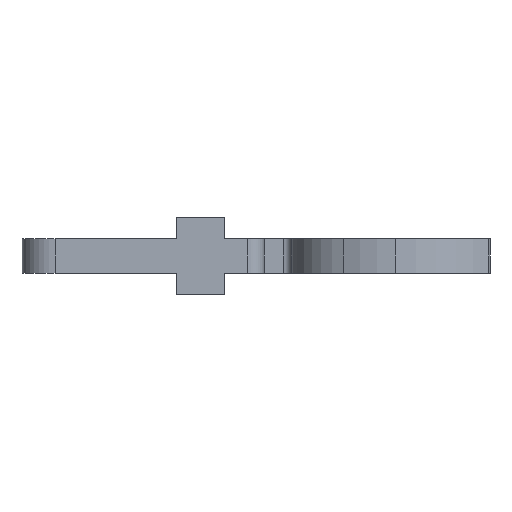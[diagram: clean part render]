
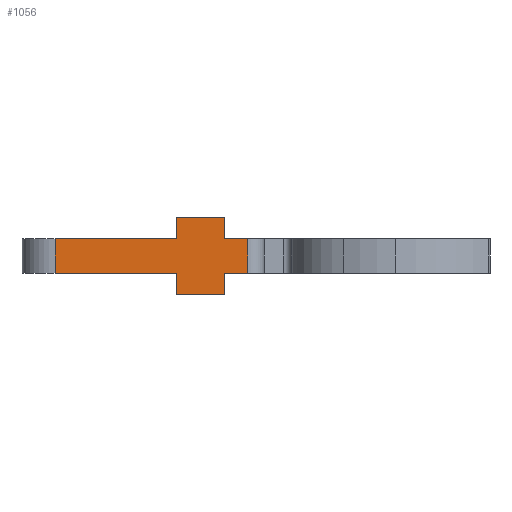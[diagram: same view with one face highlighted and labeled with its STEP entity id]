
A CAD part, left-side view. The second image highlights one B-rep face of the part: STEP entity #1056.
In plain terms, the highlighted planar face has unit normal (-1, 0, 0).
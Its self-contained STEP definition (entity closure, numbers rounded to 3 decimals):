
#2 = LINE ( 'NONE', #1489, #1785 ) ;
#8 = VERTEX_POINT ( 'NONE', #1669 ) ;
#20 = VERTEX_POINT ( 'NONE', #1665 ) ;
#34 = VERTEX_POINT ( 'NONE', #1617 ) ;
#60 = LINE ( 'NONE', #1410, #756 ) ;
#91 = LINE ( 'NONE', #1446, #873 ) ;
#95 = LINE ( 'NONE', #1477, #1276 ) ;
#170 = LINE ( 'NONE', #390, #1345 ) ;
#235 = LINE ( 'NONE', #439, #650 ) ;
#284 = EDGE_CURVE ( 'NONE', #642, #856, #235, .T. ) ;
#305 = EDGE_CURVE ( 'NONE', #1772, #20, #170, .T. ) ;
#320 = DIRECTION ( 'NONE',  ( 0., -1., 0. ) ) ;
#344 = VECTOR ( 'NONE', #1428, 1000. ) ;
#347 = VERTEX_POINT ( 'NONE', #1782 ) ;
#359 = EDGE_CURVE ( 'NONE', #765, #8, #903, .T. ) ;
#377 = VECTOR ( 'NONE', #1806, 1000. ) ;
#390 = CARTESIAN_POINT ( 'NONE',  ( 0., 23.241, 0. ) ) ;
#391 = CARTESIAN_POINT ( 'NONE',  ( 0., 20.066, 0. ) ) ;
#400 = LINE ( 'NONE', #1427, #817 ) ;
#413 = CARTESIAN_POINT ( 'NONE',  ( 0., 8.382, 3.302 ) ) ;
#439 = CARTESIAN_POINT ( 'NONE',  ( 0., 23.241, 0. ) ) ;
#441 = CARTESIAN_POINT ( 'NONE',  ( 0., 3.81, 5.334 ) ) ;
#468 = DIRECTION ( 'NONE',  ( 0., -1., 0. ) ) ;
#540 = EDGE_CURVE ( 'NONE', #856, #8, #1574, .T. ) ;
#547 = EDGE_CURVE ( 'NONE', #1663, #765, #2, .T. ) ;
#548 = EDGE_CURVE ( 'NONE', #1128, #1663, #95, .T. ) ;
#556 = EDGE_CURVE ( 'NONE', #1128, #1730, #91, .T. ) ;
#561 = EDGE_CURVE ( 'NONE', #34, #1730, #1613, .T. ) ;
#580 = EDGE_CURVE ( 'NONE', #34, #1772, #400, .T. ) ;
#583 = EDGE_CURVE ( 'NONE', #347, #20, #60, .T. ) ;
#589 = EDGE_CURVE ( 'NONE', #1293, #347, #1566, .T. ) ;
#592 = CARTESIAN_POINT ( 'NONE',  ( 0., 3.81, -2.032 ) ) ;
#593 = EDGE_CURVE ( 'NONE', #1293, #642, #1229, .T. ) ;
#642 = VERTEX_POINT ( 'NONE', #1357 ) ;
#650 = VECTOR ( 'NONE', #468, 1000. ) ;
#677 = CARTESIAN_POINT ( 'NONE',  ( 0., 8.382, 5.334 ) ) ;
#700 = DIRECTION ( 'NONE',  ( 0., 1., 0. ) ) ;
#704 = CARTESIAN_POINT ( 'NONE',  ( 0., 23.241, 3.302 ) ) ;
#714 = ORIENTED_EDGE ( 'NONE', *, *, #305, .T. ) ;
#718 = ORIENTED_EDGE ( 'NONE', *, *, #589, .F. ) ;
#729 = DIRECTION ( 'NONE',  ( 1., 0., 0. ) ) ;
#752 = PLANE ( 'NONE',  #1766 ) ;
#756 = VECTOR ( 'NONE', #1404, 1000. ) ;
#765 = VERTEX_POINT ( 'NONE', #1174 ) ;
#802 = ORIENTED_EDGE ( 'NONE', *, *, #580, .T. ) ;
#803 = ORIENTED_EDGE ( 'NONE', *, *, #561, .F. ) ;
#817 = VECTOR ( 'NONE', #1444, 1000. ) ;
#856 = VERTEX_POINT ( 'NONE', #997 ) ;
#873 = VECTOR ( 'NONE', #1457, 1000. ) ;
#903 = LINE ( 'NONE', #1817, #377 ) ;
#997 = CARTESIAN_POINT ( 'NONE',  ( 0., 1.587, 0. ) ) ;
#1007 = ORIENTED_EDGE ( 'NONE', *, *, #583, .F. ) ;
#1013 = FACE_OUTER_BOUND ( 'NONE', #1508, .T. ) ;
#1056 = ADVANCED_FACE ( 'NONE', ( #1013 ), #752, .F. ) ;
#1079 = ORIENTED_EDGE ( 'NONE', *, *, #593, .T. ) ;
#1107 = ORIENTED_EDGE ( 'NONE', *, *, #540, .T. ) ;
#1128 = VERTEX_POINT ( 'NONE', #677 ) ;
#1174 = CARTESIAN_POINT ( 'NONE',  ( 0., 3.81, 3.302 ) ) ;
#1184 = VECTOR ( 'NONE', #1396, 1000. ) ;
#1229 = LINE ( 'NONE', #1409, #1518 ) ;
#1233 = ORIENTED_EDGE ( 'NONE', *, *, #556, .T. ) ;
#1235 = VECTOR ( 'NONE', #1497, 1000. ) ;
#1276 = VECTOR ( 'NONE', #1463, 1000. ) ;
#1287 = ORIENTED_EDGE ( 'NONE', *, *, #548, .F. ) ;
#1293 = VERTEX_POINT ( 'NONE', #592 ) ;
#1305 = ORIENTED_EDGE ( 'NONE', *, *, #284, .T. ) ;
#1345 = VECTOR ( 'NONE', #320, 1000. ) ;
#1357 = CARTESIAN_POINT ( 'NONE',  ( 0., 3.81, 0. ) ) ;
#1396 = DIRECTION ( 'NONE',  ( 0., 1., 0. ) ) ;
#1403 = DIRECTION ( 'NONE',  ( 0., 0., 1. ) ) ;
#1404 = DIRECTION ( 'NONE',  ( 0., 0., 1. ) ) ;
#1406 = ORIENTED_EDGE ( 'NONE', *, *, #359, .F. ) ;
#1409 = CARTESIAN_POINT ( 'NONE',  ( 0., 3.81, -2.032 ) ) ;
#1410 = CARTESIAN_POINT ( 'NONE',  ( 0., 8.382, -2.032 ) ) ;
#1427 = CARTESIAN_POINT ( 'NONE',  ( 0., 20.066, 3.302 ) ) ;
#1428 = DIRECTION ( 'NONE',  ( 0., -1., 0. ) ) ;
#1432 = CARTESIAN_POINT ( 'NONE',  ( 0., 8.382, -2.032 ) ) ;
#1435 = CARTESIAN_POINT ( 'NONE',  ( 0., 23.241, 3.302 ) ) ;
#1444 = DIRECTION ( 'NONE',  ( 0., 0., -1. ) ) ;
#1446 = CARTESIAN_POINT ( 'NONE',  ( 0., 8.382, 5.334 ) ) ;
#1457 = DIRECTION ( 'NONE',  ( 0., 0., -1. ) ) ;
#1463 = DIRECTION ( 'NONE',  ( 0., -1., 0. ) ) ;
#1472 = DIRECTION ( 'NONE',  ( 0., 0., -1. ) ) ;
#1477 = CARTESIAN_POINT ( 'NONE',  ( 0., 3.81, 5.334 ) ) ;
#1489 = CARTESIAN_POINT ( 'NONE',  ( 0., 3.81, 5.334 ) ) ;
#1496 = CARTESIAN_POINT ( 'NONE',  ( 0., 1.587, 3.302 ) ) ;
#1497 = DIRECTION ( 'NONE',  ( 0., 0., 1. ) ) ;
#1508 = EDGE_LOOP ( 'NONE', ( #1305, #1107, #1406, #1801, #1287, #1233, #803, #802, #714, #1007, #718, #1079 ) ) ;
#1518 = VECTOR ( 'NONE', #1403, 1000. ) ;
#1566 = LINE ( 'NONE', #1432, #1184 ) ;
#1574 = LINE ( 'NONE', #1496, #1235 ) ;
#1613 = LINE ( 'NONE', #1435, #344 ) ;
#1617 = CARTESIAN_POINT ( 'NONE',  ( 0., 20.066, 3.302 ) ) ;
#1663 = VERTEX_POINT ( 'NONE', #441 ) ;
#1665 = CARTESIAN_POINT ( 'NONE',  ( 0., 8.382, 0. ) ) ;
#1669 = CARTESIAN_POINT ( 'NONE',  ( 0., 1.587, 3.302 ) ) ;
#1730 = VERTEX_POINT ( 'NONE', #413 ) ;
#1766 = AXIS2_PLACEMENT_3D ( 'NONE', #704, #729, #700 ) ;
#1772 = VERTEX_POINT ( 'NONE', #391 ) ;
#1782 = CARTESIAN_POINT ( 'NONE',  ( 0., 8.382, -2.032 ) ) ;
#1785 = VECTOR ( 'NONE', #1472, 1000. ) ;
#1801 = ORIENTED_EDGE ( 'NONE', *, *, #547, .F. ) ;
#1806 = DIRECTION ( 'NONE',  ( 0., -1., 0. ) ) ;
#1817 = CARTESIAN_POINT ( 'NONE',  ( 0., 23.241, 3.302 ) ) ;
